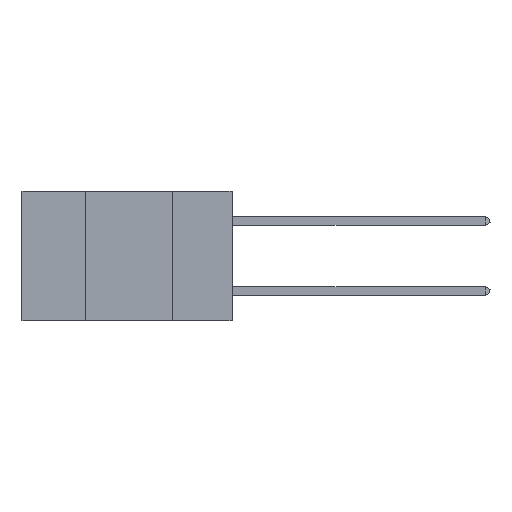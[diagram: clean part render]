
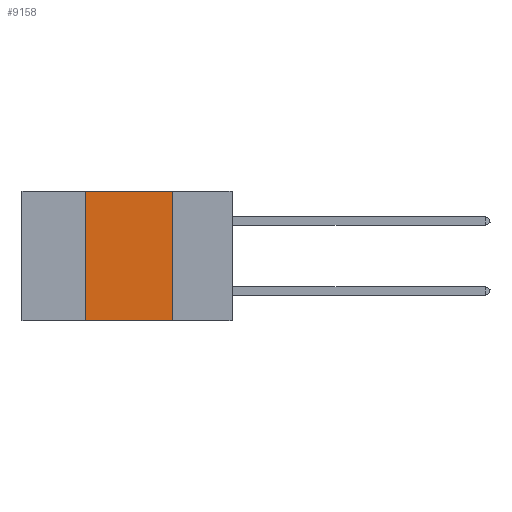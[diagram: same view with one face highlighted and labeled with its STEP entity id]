
A CAD part, left-side view. The second image highlights one B-rep face of the part: STEP entity #9158.
In plain terms, the highlighted planar face has unit normal (-1, 0, 0).
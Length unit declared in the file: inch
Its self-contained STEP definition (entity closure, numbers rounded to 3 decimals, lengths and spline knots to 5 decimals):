
#1359 = CARTESIAN_POINT ( 'NONE',  ( 0., 0.17, 0. ) ) ;
#1844 = EDGE_LOOP ( 'NONE', ( #11503, #20304, #6819, #17272 ) ) ;
#2684 = CARTESIAN_POINT ( 'NONE',  ( 0., 0.42, 0. ) ) ;
#2809 = LINE ( 'NONE', #2684, #7346 ) ;
#2844 = VERTEX_POINT ( 'NONE', #21409 ) ;
#3614 = CARTESIAN_POINT ( 'NONE',  ( 0., 0.6, 0. ) ) ;
#4249 = FACE_OUTER_BOUND ( 'NONE', #1844, .T. ) ;
#4534 = EDGE_CURVE ( 'NONE', #20278, #9622, #18769, .T. ) ;
#5004 = VECTOR ( 'NONE', #14646, 39.37008 ) ;
#5354 = DIRECTION ( 'NONE',  ( 1., 0., 0. ) ) ;
#5484 = VECTOR ( 'NONE', #17168, 39.37008 ) ;
#6771 = DIRECTION ( 'NONE',  ( 0., 0., -1. ) ) ;
#6819 = ORIENTED_EDGE ( 'NONE', *, *, #20566, .F. ) ;
#7346 = VECTOR ( 'NONE', #14455, 39.37008 ) ;
#8190 = VECTOR ( 'NONE', #6771, 39.37008 ) ;
#8982 = CARTESIAN_POINT ( 'NONE',  ( 0., 0.42, -0.37 ) ) ;
#9158 = ADVANCED_FACE ( 'NONE', ( #4249 ), #15325, .F. ) ;
#9622 = VERTEX_POINT ( 'NONE', #1359 ) ;
#9915 = CARTESIAN_POINT ( 'NONE',  ( 0., 0.42, 0. ) ) ;
#10205 = EDGE_CURVE ( 'NONE', #14038, #2844, #19333, .T. ) ;
#11503 = ORIENTED_EDGE ( 'NONE', *, *, #19187, .F. ) ;
#13906 = CARTESIAN_POINT ( 'NONE',  ( 0., 0.6, 0. ) ) ;
#14038 = VERTEX_POINT ( 'NONE', #8982 ) ;
#14455 = DIRECTION ( 'NONE',  ( 0., 0., 1. ) ) ;
#14646 = DIRECTION ( 'NONE',  ( 0., -1., 0. ) ) ;
#15070 = CARTESIAN_POINT ( 'NONE',  ( 0., 0.17, 0. ) ) ;
#15325 = PLANE ( 'NONE',  #18223 ) ;
#17002 = DIRECTION ( 'NONE',  ( 0., 0., -1. ) ) ;
#17168 = DIRECTION ( 'NONE',  ( 0., -1., 0. ) ) ;
#17272 = ORIENTED_EDGE ( 'NONE', *, *, #10205, .T. ) ;
#18223 = AXIS2_PLACEMENT_3D ( 'NONE', #3614, #5354, #17002 ) ;
#18769 = LINE ( 'NONE', #13906, #5484 ) ;
#19187 = EDGE_CURVE ( 'NONE', #9622, #2844, #21385, .T. ) ;
#19333 = LINE ( 'NONE', #19555, #5004 ) ;
#19555 = CARTESIAN_POINT ( 'NONE',  ( 0., 0.6, -0.37 ) ) ;
#20278 = VERTEX_POINT ( 'NONE', #9915 ) ;
#20304 = ORIENTED_EDGE ( 'NONE', *, *, #4534, .F. ) ;
#20566 = EDGE_CURVE ( 'NONE', #14038, #20278, #2809, .T. ) ;
#21385 = LINE ( 'NONE', #15070, #8190 ) ;
#21409 = CARTESIAN_POINT ( 'NONE',  ( 0., 0.17, -0.37 ) ) ;
